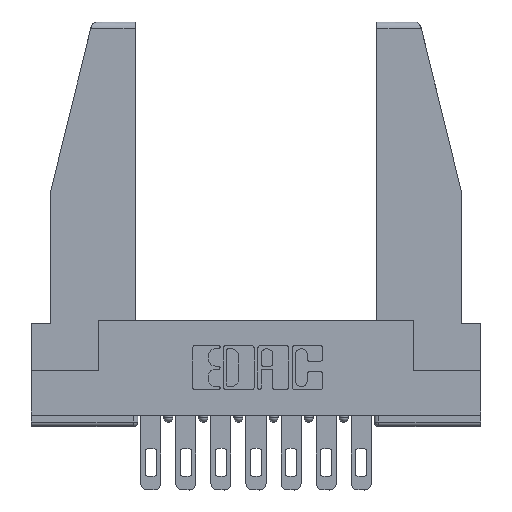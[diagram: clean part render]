
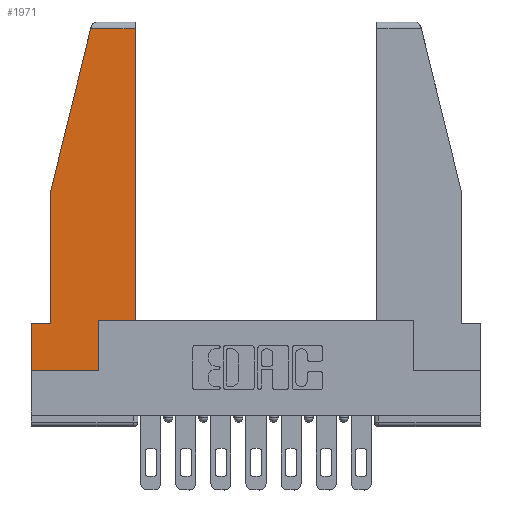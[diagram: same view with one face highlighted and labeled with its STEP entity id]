
A CAD part, top view. The second image highlights one B-rep face of the part: STEP entity #1971.
In plain terms, the highlighted planar face has unit normal (0, 0, 1).
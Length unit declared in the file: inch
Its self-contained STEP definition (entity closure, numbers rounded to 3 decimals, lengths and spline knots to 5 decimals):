
#61 = CARTESIAN_POINT ( 'NONE',  ( 0., 0., 0. ) ) ;
#81 = CARTESIAN_POINT ( 'NONE',  ( 0., 0., 0. ) ) ;
#139 = CARTESIAN_POINT ( 'NONE',  ( 0.086, 0.8, 0. ) ) ;
#265 = ORIENTED_EDGE ( 'NONE', *, *, #10166, .T. ) ;
#451 = EDGE_CURVE ( 'NONE', #12168, #8549, #11415, .T. ) ;
#493 = CARTESIAN_POINT ( 'NONE',  ( 0., 0.21, 0. ) ) ;
#1619 = VECTOR ( 'NONE', #5563, 39.37008 ) ;
#1700 = DIRECTION ( 'NONE',  ( 1., 0., 0. ) ) ;
#1808 = LINE ( 'NONE', #5034, #10567 ) ;
#1917 = ORIENTED_EDGE ( 'NONE', *, *, #9784, .T. ) ;
#1971 = ADVANCED_FACE ( 'NONE', ( #11553 ), #11905, .T. ) ;
#2136 = DIRECTION ( 'NONE',  ( 1., 0., 0. ) ) ;
#2215 = ORIENTED_EDGE ( 'NONE', *, *, #3530, .T. ) ;
#2253 = DIRECTION ( 'NONE',  ( -0.239, -0.971, 0. ) ) ;
#2522 = CARTESIAN_POINT ( 'NONE',  ( 0.461, 0.223, 0. ) ) ;
#2676 = VERTEX_POINT ( 'NONE', #9401 ) ;
#2724 = CARTESIAN_POINT ( 'NONE',  ( 0.297, 0., 0. ) ) ;
#3096 = ORIENTED_EDGE ( 'NONE', *, *, #3827, .T. ) ;
#3250 = DIRECTION ( 'NONE',  ( -1., 0., 0. ) ) ;
#3459 = LINE ( 'NONE', #12407, #8686 ) ;
#3526 = LINE ( 'NONE', #8234, #9228 ) ;
#3530 = EDGE_CURVE ( 'NONE', #4526, #10674, #3526, .T. ) ;
#3765 = VERTEX_POINT ( 'NONE', #8978 ) ;
#3827 = EDGE_CURVE ( 'NONE', #2676, #4526, #1808, .T. ) ;
#3981 = VERTEX_POINT ( 'NONE', #2724 ) ;
#4002 = VERTEX_POINT ( 'NONE', #11577 ) ;
#4526 = VERTEX_POINT ( 'NONE', #6513 ) ;
#4732 = VECTOR ( 'NONE', #7933, 39.37008 ) ;
#4924 = DIRECTION ( 'NONE',  ( 1., 0., 0. ) ) ;
#4942 = ORIENTED_EDGE ( 'NONE', *, *, #10991, .T. ) ;
#5034 = CARTESIAN_POINT ( 'NONE',  ( 0., 1.52, 0. ) ) ;
#5563 = DIRECTION ( 'NONE',  ( 0., -1., 0. ) ) ;
#5771 = VECTOR ( 'NONE', #1700, 39.37008 ) ;
#5772 = DIRECTION ( 'NONE',  ( 0., -1., 0. ) ) ;
#5829 = EDGE_CURVE ( 'NONE', #6506, #3981, #11887, .T. ) ;
#5953 = LINE ( 'NONE', #9454, #1619 ) ;
#6370 = CARTESIAN_POINT ( 'NONE',  ( 0.297, 0.223, 0. ) ) ;
#6506 = VERTEX_POINT ( 'NONE', #7142 ) ;
#6513 = CARTESIAN_POINT ( 'NONE',  ( 0.2636, 1.52, 0. ) ) ;
#6897 = CARTESIAN_POINT ( 'NONE',  ( 0.297, 0., 0. ) ) ;
#7142 = CARTESIAN_POINT ( 'NONE',  ( 0., 0., 0. ) ) ;
#7699 = DIRECTION ( 'NONE',  ( 0., 0., 1. ) ) ;
#7767 = ORIENTED_EDGE ( 'NONE', *, *, #12214, .T. ) ;
#7802 = ORIENTED_EDGE ( 'NONE', *, *, #451, .T. ) ;
#7933 = DIRECTION ( 'NONE',  ( -1., 0., 0. ) ) ;
#8234 = CARTESIAN_POINT ( 'NONE',  ( 0.271, 1.55, 0. ) ) ;
#8397 = ORIENTED_EDGE ( 'NONE', *, *, #10523, .T. ) ;
#8549 = VERTEX_POINT ( 'NONE', #2522 ) ;
#8681 = LINE ( 'NONE', #493, #9154 ) ;
#8686 = VECTOR ( 'NONE', #9387, 39.37008 ) ;
#8776 = ORIENTED_EDGE ( 'NONE', *, *, #5829, .T. ) ;
#8978 = CARTESIAN_POINT ( 'NONE',  ( 0.086, 0.21, 0. ) ) ;
#9039 = LINE ( 'NONE', #11890, #4732 ) ;
#9154 = VECTOR ( 'NONE', #5772, 39.37008 ) ;
#9177 = VECTOR ( 'NONE', #11830, 39.37008 ) ;
#9228 = VECTOR ( 'NONE', #2253, 39.37008 ) ;
#9387 = DIRECTION ( 'NONE',  ( 0., 1., 0. ) ) ;
#9401 = CARTESIAN_POINT ( 'NONE',  ( 0.461, 1.52, 0. ) ) ;
#9454 = CARTESIAN_POINT ( 'NONE',  ( 0.086, 0.8, 0. ) ) ;
#9619 = EDGE_LOOP ( 'NONE', ( #4942, #3096, #2215, #1917, #265, #7767, #8776, #8397, #7802 ) ) ;
#9784 = EDGE_CURVE ( 'NONE', #10674, #3765, #5953, .T. ) ;
#10166 = EDGE_CURVE ( 'NONE', #3765, #4002, #9039, .T. ) ;
#10402 = AXIS2_PLACEMENT_3D ( 'NONE', #81, #7699, #4924 ) ;
#10523 = EDGE_CURVE ( 'NONE', #3981, #12168, #11449, .T. ) ;
#10567 = VECTOR ( 'NONE', #3250, 39.37008 ) ;
#10674 = VERTEX_POINT ( 'NONE', #139 ) ;
#10991 = EDGE_CURVE ( 'NONE', #8549, #2676, #3459, .T. ) ;
#11415 = LINE ( 'NONE', #11548, #5771 ) ;
#11449 = LINE ( 'NONE', #6897, #9177 ) ;
#11548 = CARTESIAN_POINT ( 'NONE',  ( 0.297, 0.223, 0. ) ) ;
#11553 = FACE_OUTER_BOUND ( 'NONE', #9619, .T. ) ;
#11577 = CARTESIAN_POINT ( 'NONE',  ( 0., 0.21, 0. ) ) ;
#11830 = DIRECTION ( 'NONE',  ( 0., 1., 0. ) ) ;
#11887 = LINE ( 'NONE', #61, #12213 ) ;
#11890 = CARTESIAN_POINT ( 'NONE',  ( 0., 0.21, 0. ) ) ;
#11905 = PLANE ( 'NONE',  #10402 ) ;
#12168 = VERTEX_POINT ( 'NONE', #6370 ) ;
#12213 = VECTOR ( 'NONE', #2136, 39.37008 ) ;
#12214 = EDGE_CURVE ( 'NONE', #4002, #6506, #8681, .T. ) ;
#12407 = CARTESIAN_POINT ( 'NONE',  ( 0.461, 0.223, 0. ) ) ;
